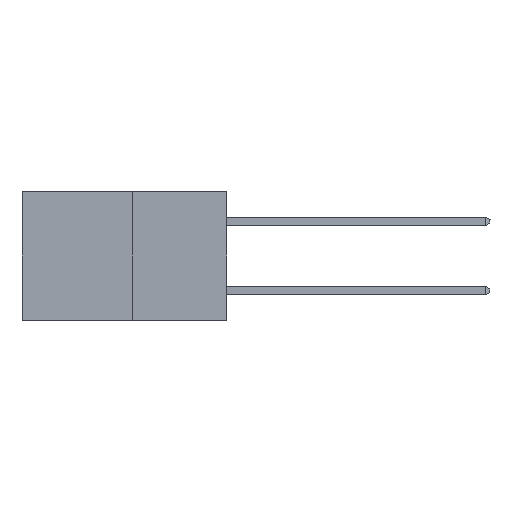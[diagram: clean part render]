
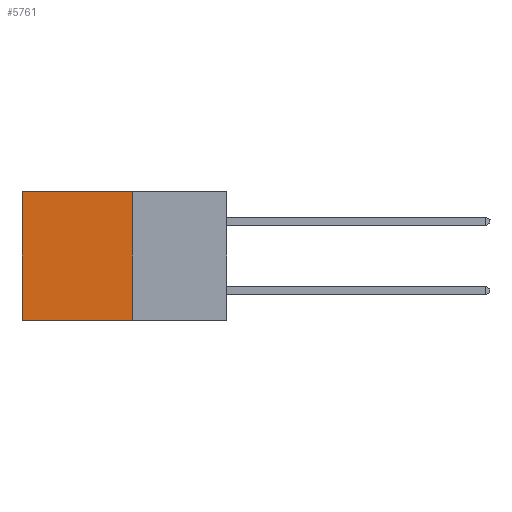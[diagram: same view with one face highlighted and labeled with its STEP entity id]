
A CAD part, left-side view. The second image highlights one B-rep face of the part: STEP entity #5761.
In plain terms, the highlighted planar face has unit normal (-1, 0, 0).
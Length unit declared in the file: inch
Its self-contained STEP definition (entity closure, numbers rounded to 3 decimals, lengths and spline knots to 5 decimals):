
#265 = ORIENTED_EDGE ( 'NONE', *, *, #13034, .F. ) ;
#819 = CARTESIAN_POINT ( 'NONE',  ( 0.277, 0.27, 0. ) ) ;
#2094 = EDGE_CURVE ( 'NONE', #13030, #14564, #2835, .T. ) ;
#2097 = VECTOR ( 'NONE', #11971, 39.37008 ) ;
#2449 = VECTOR ( 'NONE', #8505, 39.37008 ) ;
#2835 = LINE ( 'NONE', #8968, #2449 ) ;
#3397 = EDGE_CURVE ( 'NONE', #3551, #6016, #12694, .T. ) ;
#3551 = VERTEX_POINT ( 'NONE', #10214 ) ;
#4133 = ORIENTED_EDGE ( 'NONE', *, *, #3397, .T. ) ;
#4137 = DIRECTION ( 'NONE',  ( 0., 0., -1. ) ) ;
#4573 = EDGE_CURVE ( 'NONE', #6016, #14564, #5392, .T. ) ;
#4974 = FACE_OUTER_BOUND ( 'NONE', #7989, .T. ) ;
#5334 = CARTESIAN_POINT ( 'NONE',  ( 0.277, 0.27, -0.37 ) ) ;
#5392 = LINE ( 'NONE', #7176, #2097 ) ;
#5671 = ORIENTED_EDGE ( 'NONE', *, *, #2094, .F. ) ;
#5761 = ADVANCED_FACE ( 'NONE', ( #4974 ), #13808, .F. ) ;
#6016 = VERTEX_POINT ( 'NONE', #7585 ) ;
#6524 = AXIS2_PLACEMENT_3D ( 'NONE', #13738, #10079, #10105 ) ;
#7176 = CARTESIAN_POINT ( 'NONE',  ( 0.277, 0.59, -0.37 ) ) ;
#7585 = CARTESIAN_POINT ( 'NONE',  ( 0.277, 0.59, 0. ) ) ;
#7989 = EDGE_LOOP ( 'NONE', ( #10335, #5671, #265, #4133 ) ) ;
#8468 = VECTOR ( 'NONE', #4137, 39.37008 ) ;
#8505 = DIRECTION ( 'NONE',  ( 0., 1., 0. ) ) ;
#8968 = CARTESIAN_POINT ( 'NONE',  ( 0.277, 0.27, -0.37 ) ) ;
#9734 = VECTOR ( 'NONE', #12509, 39.37008 ) ;
#10079 = DIRECTION ( 'NONE',  ( 1., 0., 0. ) ) ;
#10105 = DIRECTION ( 'NONE',  ( 0., 0., -1. ) ) ;
#10214 = CARTESIAN_POINT ( 'NONE',  ( 0.277, 0.27, 0. ) ) ;
#10335 = ORIENTED_EDGE ( 'NONE', *, *, #4573, .T. ) ;
#11971 = DIRECTION ( 'NONE',  ( 0., 0., -1. ) ) ;
#12509 = DIRECTION ( 'NONE',  ( 0., 1., 0. ) ) ;
#12694 = LINE ( 'NONE', #819, #9734 ) ;
#13030 = VERTEX_POINT ( 'NONE', #5334 ) ;
#13034 = EDGE_CURVE ( 'NONE', #3551, #13030, #14442, .T. ) ;
#13232 = CARTESIAN_POINT ( 'NONE',  ( 0.277, 0.27, -0.37 ) ) ;
#13738 = CARTESIAN_POINT ( 'NONE',  ( 0.277, 0.27, -0.37 ) ) ;
#13808 = PLANE ( 'NONE',  #6524 ) ;
#14249 = CARTESIAN_POINT ( 'NONE',  ( 0.277, 0.59, -0.37 ) ) ;
#14442 = LINE ( 'NONE', #13232, #8468 ) ;
#14564 = VERTEX_POINT ( 'NONE', #14249 ) ;
